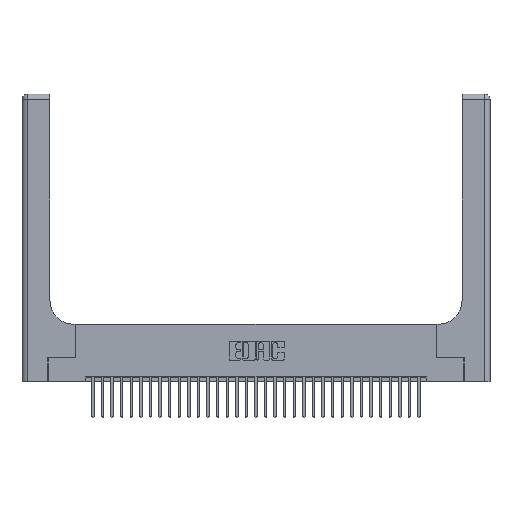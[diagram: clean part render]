
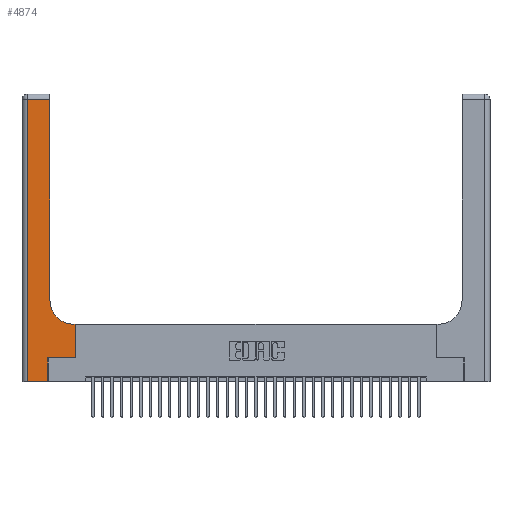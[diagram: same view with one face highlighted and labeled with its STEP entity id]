
A CAD part, top view. The second image highlights one B-rep face of the part: STEP entity #4874.
In plain terms, the highlighted planar face has unit normal (0, 0, 1).
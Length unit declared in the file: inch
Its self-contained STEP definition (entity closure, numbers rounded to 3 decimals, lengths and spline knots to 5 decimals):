
#286 = VERTEX_POINT ( 'NONE', #8473 ) ;
#991 = DIRECTION ( 'NONE',  ( 0., 0., -1. ) ) ;
#1080 = VERTEX_POINT ( 'NONE', #7854 ) ;
#1136 = AXIS2_PLACEMENT_3D ( 'NONE', #22972, #15396, #33376 ) ;
#1370 = CARTESIAN_POINT ( 'NONE',  ( 0., 2.94, 0.37 ) ) ;
#1431 = EDGE_CURVE ( 'NONE', #28832, #15121, #27117, .T. ) ;
#2299 = DIRECTION ( 'NONE',  ( 1., 0., 0. ) ) ;
#2483 = VECTOR ( 'NONE', #9789, 39.37008 ) ;
#2801 = VECTOR ( 'NONE', #19006, 39.37008 ) ;
#3293 = LINE ( 'NONE', #32924, #2483 ) ;
#3985 = DIRECTION ( 'NONE',  ( -1., 0., 0. ) ) ;
#4192 = CARTESIAN_POINT ( 'NONE',  ( 0.5585, 0.25, 0.37 ) ) ;
#4654 = VERTEX_POINT ( 'NONE', #11869 ) ;
#4874 = ADVANCED_FACE ( 'NONE', ( #15763 ), #12773, .F. ) ;
#5228 = CARTESIAN_POINT ( 'NONE',  ( 0.06, 0., 0.37 ) ) ;
#6470 = VECTOR ( 'NONE', #3985, 39.37008 ) ;
#7191 = EDGE_CURVE ( 'NONE', #1080, #286, #10689, .T. ) ;
#7480 = ORIENTED_EDGE ( 'NONE', *, *, #21085, .T. ) ;
#7831 = DIRECTION ( 'NONE',  ( 1., 0., 0. ) ) ;
#7854 = CARTESIAN_POINT ( 'NONE',  ( 0.5585, 0.6, 0.37 ) ) ;
#8473 = CARTESIAN_POINT ( 'NONE',  ( 0.5415, 0.6, 0.37 ) ) ;
#8660 = VECTOR ( 'NONE', #14673, 39.37008 ) ;
#9142 = ORIENTED_EDGE ( 'NONE', *, *, #24355, .T. ) ;
#9315 = CARTESIAN_POINT ( 'NONE',  ( 0.2915, 2.94, 0.37 ) ) ;
#9789 = DIRECTION ( 'NONE',  ( 0., -1., 0. ) ) ;
#10342 = EDGE_LOOP ( 'NONE', ( #28210, #23352, #32228, #24936, #14067, #9142, #7480, #11112, #26398 ) ) ;
#10689 = LINE ( 'NONE', #21432, #2801 ) ;
#11112 = ORIENTED_EDGE ( 'NONE', *, *, #7191, .T. ) ;
#11869 = CARTESIAN_POINT ( 'NONE',  ( 0.269, 0.25, 0.37 ) ) ;
#12363 = CARTESIAN_POINT ( 'NONE',  ( 0.06, 2.94, 0.37 ) ) ;
#12773 = PLANE ( 'NONE',  #1136 ) ;
#14067 = ORIENTED_EDGE ( 'NONE', *, *, #25376, .T. ) ;
#14221 = VECTOR ( 'NONE', #7831, 39.37008 ) ;
#14673 = DIRECTION ( 'NONE',  ( 0., 1., 0. ) ) ;
#14786 = VECTOR ( 'NONE', #22402, 39.37008 ) ;
#14931 = EDGE_CURVE ( 'NONE', #30646, #28832, #27962, .T. ) ;
#15121 = VERTEX_POINT ( 'NONE', #12363 ) ;
#15396 = DIRECTION ( 'NONE',  ( 0., 0., -1. ) ) ;
#15633 = LINE ( 'NONE', #27420, #8660 ) ;
#15637 = CARTESIAN_POINT ( 'NONE',  ( 0., 0., 0.37 ) ) ;
#15763 = FACE_OUTER_BOUND ( 'NONE', #10342, .T. ) ;
#16513 = CARTESIAN_POINT ( 'NONE',  ( 0.269, 0., 0.37 ) ) ;
#16581 = CARTESIAN_POINT ( 'NONE',  ( 0.2915, 3., 0.37 ) ) ;
#16707 = CARTESIAN_POINT ( 'NONE',  ( 0.5415, 0.85, 0.37 ) ) ;
#19006 = DIRECTION ( 'NONE',  ( -1., 0., 0. ) ) ;
#19282 = DIRECTION ( 'NONE',  ( 1., 0., 0. ) ) ;
#20247 = CARTESIAN_POINT ( 'NONE',  ( 0.5585, 0.25, 0.37 ) ) ;
#20350 = VECTOR ( 'NONE', #26830, 39.37008 ) ;
#21031 = LINE ( 'NONE', #15637, #14221 ) ;
#21085 = EDGE_CURVE ( 'NONE', #27603, #1080, #27590, .T. ) ;
#21432 = CARTESIAN_POINT ( 'NONE',  ( 0.2915, 0.6, 0.37 ) ) ;
#22402 = DIRECTION ( 'NONE',  ( 0., 1., 0. ) ) ;
#22972 = CARTESIAN_POINT ( 'NONE',  ( 0., 3., 0.37 ) ) ;
#23352 = ORIENTED_EDGE ( 'NONE', *, *, #1431, .T. ) ;
#24355 = EDGE_CURVE ( 'NONE', #4654, #27603, #25742, .T. ) ;
#24910 = EDGE_CURVE ( 'NONE', #15121, #31065, #3293, .T. ) ;
#24936 = ORIENTED_EDGE ( 'NONE', *, *, #28432, .T. ) ;
#24943 = VECTOR ( 'NONE', #2299, 39.37008 ) ;
#25376 = EDGE_CURVE ( 'NONE', #32478, #4654, #15633, .T. ) ;
#25742 = LINE ( 'NONE', #33403, #24943 ) ;
#25867 = AXIS2_PLACEMENT_3D ( 'NONE', #16707, #991, #19282 ) ;
#26398 = ORIENTED_EDGE ( 'NONE', *, *, #27315, .T. ) ;
#26830 = DIRECTION ( 'NONE',  ( 0., 1., 0. ) ) ;
#26875 = CARTESIAN_POINT ( 'NONE',  ( 0.2915, 0.85, 0.37 ) ) ;
#27117 = LINE ( 'NONE', #1370, #6470 ) ;
#27315 = EDGE_CURVE ( 'NONE', #286, #30646, #33178, .T. ) ;
#27420 = CARTESIAN_POINT ( 'NONE',  ( 0.269, 0., 0.37 ) ) ;
#27590 = LINE ( 'NONE', #4192, #14786 ) ;
#27603 = VERTEX_POINT ( 'NONE', #20247 ) ;
#27962 = LINE ( 'NONE', #16581, #20350 ) ;
#28210 = ORIENTED_EDGE ( 'NONE', *, *, #14931, .T. ) ;
#28432 = EDGE_CURVE ( 'NONE', #31065, #32478, #21031, .T. ) ;
#28832 = VERTEX_POINT ( 'NONE', #9315 ) ;
#30646 = VERTEX_POINT ( 'NONE', #26875 ) ;
#31065 = VERTEX_POINT ( 'NONE', #5228 ) ;
#32228 = ORIENTED_EDGE ( 'NONE', *, *, #24910, .T. ) ;
#32478 = VERTEX_POINT ( 'NONE', #16513 ) ;
#32924 = CARTESIAN_POINT ( 'NONE',  ( 0.06, 3., 0.37 ) ) ;
#33178 = CIRCLE ( 'NONE', #25867, 0.25 ) ;
#33376 = DIRECTION ( 'NONE',  ( -1., 0., 0. ) ) ;
#33403 = CARTESIAN_POINT ( 'NONE',  ( 0.269, 0.25, 0.37 ) ) ;
